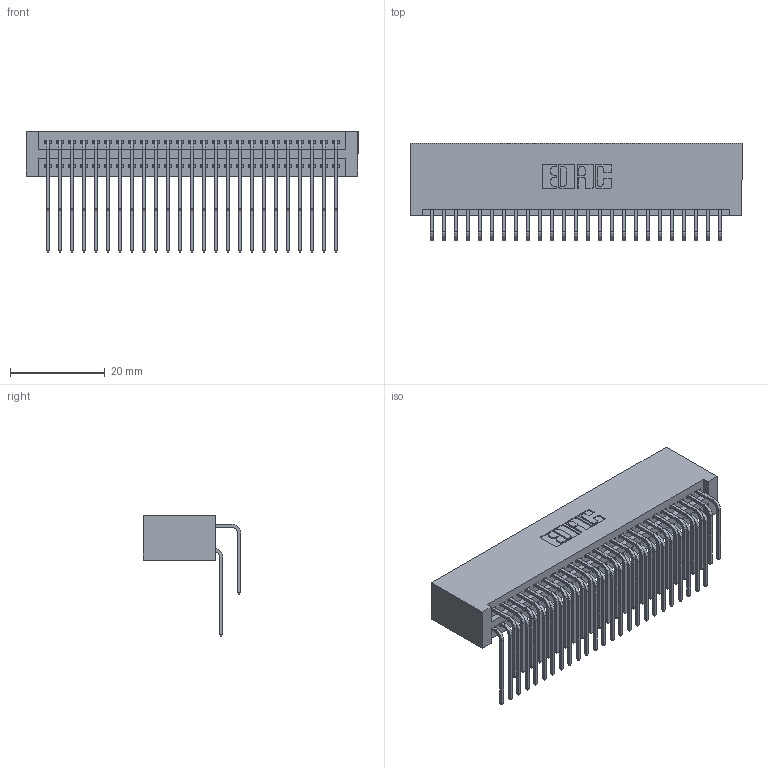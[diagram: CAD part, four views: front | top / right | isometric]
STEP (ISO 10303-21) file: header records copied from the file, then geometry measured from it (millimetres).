
FILE_DESCRIPTION (( 'STEP AP203' ), '1' );
FILE_NAME ('395-050-559-201.STEP', '2019-10-19T14:15:21', ( '' ), ( '' ), 'SwSTEP 2.0', 'SolidWorks 2016', '' );
FILE_SCHEMA (( 'CONFIG_CONTROL_DESIGN' ));
Length unit declared in the file: inch
Products named in the file (4): 345-292-001_559 Tail - 2; 395-050-559-201; 345 Part_No Mounting Lugs; 345-292-001_558 559 Tail - 1
Assembly tree (51 placements, depth 2):
  395-050-559-201
    345 Part_No Mounting Lugs
    345-292-001_558 559 Tail - 1  x25
    345-292-001_559 Tail - 2  x25
Bounding box: 70.1 x 20.56 x 25.53 mm (x, y, z)
Volume: 7556.5 mm3; surface area: 12500.1 mm2
Topology: 51 solids, 51 shells, 2718 faces, 8067 edges, 5310 vertices
Faces by surface type: plane 1826, cylinder 892
Entity records: 23279 total; most frequent: CARTESIAN_POINT 3963, ORIENTED_EDGE 3846, DIRECTION 3483, EDGE_CURVE 1923, LINE 1659, VECTOR 1659, VERTEX_POINT 1278, AXIS2_PLACEMENT_3D 912
